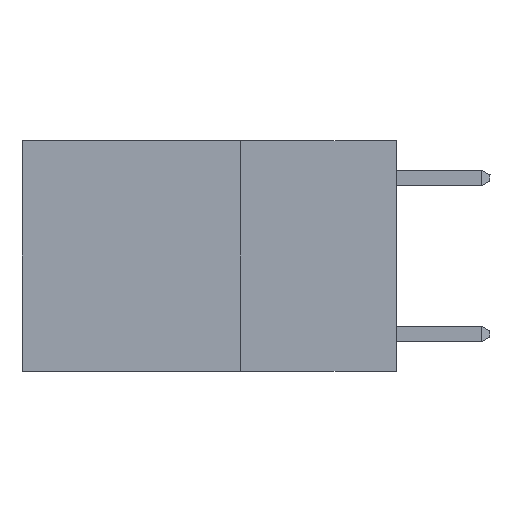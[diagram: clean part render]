
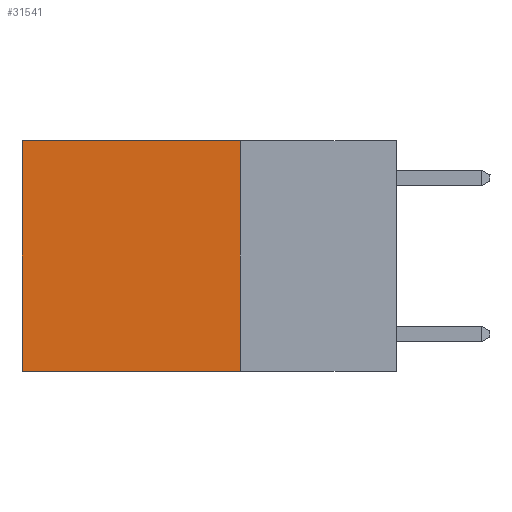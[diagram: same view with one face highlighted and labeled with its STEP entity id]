
A CAD part, left-side view. The second image highlights one B-rep face of the part: STEP entity #31541.
In plain terms, the highlighted planar face has unit normal (-1, 0, 0).
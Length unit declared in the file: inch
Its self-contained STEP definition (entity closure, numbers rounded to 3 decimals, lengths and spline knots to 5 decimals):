
#816 = PLANE ( 'NONE',  #17449 ) ;
#923 = VECTOR ( 'NONE', #18710, 39.37008 ) ;
#1260 = CARTESIAN_POINT ( 'NONE',  ( 0.2625, 0.25, -0.37 ) ) ;
#1906 = LINE ( 'NONE', #1260, #12899 ) ;
#2481 = CARTESIAN_POINT ( 'NONE',  ( 0.2625, 0.25, 0. ) ) ;
#6868 = CARTESIAN_POINT ( 'NONE',  ( 0.2625, 0.6, -0.37 ) ) ;
#7774 = ORIENTED_EDGE ( 'NONE', *, *, #18705, .T. ) ;
#8083 = DIRECTION ( 'NONE',  ( 1., 0., 0. ) ) ;
#9599 = VECTOR ( 'NONE', #20186, 39.37008 ) ;
#10972 = CARTESIAN_POINT ( 'NONE',  ( 0.2625, 0.25, 0. ) ) ;
#11374 = DIRECTION ( 'NONE',  ( 0., 0., -1. ) ) ;
#12285 = VERTEX_POINT ( 'NONE', #12782 ) ;
#12782 = CARTESIAN_POINT ( 'NONE',  ( 0.2625, 0.6, 0. ) ) ;
#12852 = EDGE_CURVE ( 'NONE', #21952, #18796, #1906, .T. ) ;
#12899 = VECTOR ( 'NONE', #20907, 39.37008 ) ;
#13937 = LINE ( 'NONE', #28430, #27181 ) ;
#14035 = LINE ( 'NONE', #26280, #923 ) ;
#14730 = EDGE_LOOP ( 'NONE', ( #7774, #15000, #30863, #27193 ) ) ;
#15000 = ORIENTED_EDGE ( 'NONE', *, *, #12852, .F. ) ;
#15680 = EDGE_CURVE ( 'NONE', #28122, #21952, #26096, .T. ) ;
#17449 = AXIS2_PLACEMENT_3D ( 'NONE', #10972, #8083, #23036 ) ;
#18705 = EDGE_CURVE ( 'NONE', #12285, #18796, #13937, .T. ) ;
#18710 = DIRECTION ( 'NONE',  ( 0., 1., 0. ) ) ;
#18796 = VERTEX_POINT ( 'NONE', #6868 ) ;
#20186 = DIRECTION ( 'NONE',  ( 0., 0., -1. ) ) ;
#20211 = CARTESIAN_POINT ( 'NONE',  ( 0.2625, 0.25, -0.37 ) ) ;
#20907 = DIRECTION ( 'NONE',  ( 0., 1., 0. ) ) ;
#21952 = VERTEX_POINT ( 'NONE', #20211 ) ;
#23036 = DIRECTION ( 'NONE',  ( 0., 0., -1. ) ) ;
#26096 = LINE ( 'NONE', #2481, #9599 ) ;
#26280 = CARTESIAN_POINT ( 'NONE',  ( 0.2625, 0.25, 0. ) ) ;
#27181 = VECTOR ( 'NONE', #11374, 39.37008 ) ;
#27193 = ORIENTED_EDGE ( 'NONE', *, *, #29870, .T. ) ;
#28122 = VERTEX_POINT ( 'NONE', #28538 ) ;
#28430 = CARTESIAN_POINT ( 'NONE',  ( 0.2625, 0.6, 0. ) ) ;
#28538 = CARTESIAN_POINT ( 'NONE',  ( 0.2625, 0.25, 0. ) ) ;
#29870 = EDGE_CURVE ( 'NONE', #28122, #12285, #14035, .T. ) ;
#30091 = FACE_OUTER_BOUND ( 'NONE', #14730, .T. ) ;
#30863 = ORIENTED_EDGE ( 'NONE', *, *, #15680, .F. ) ;
#31541 = ADVANCED_FACE ( 'NONE', ( #30091 ), #816, .F. ) ;
